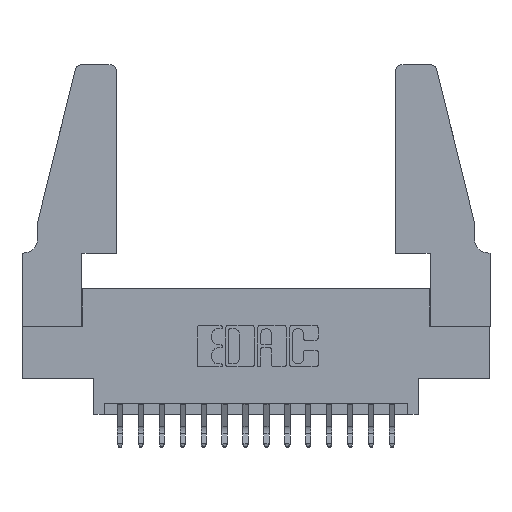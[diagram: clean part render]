
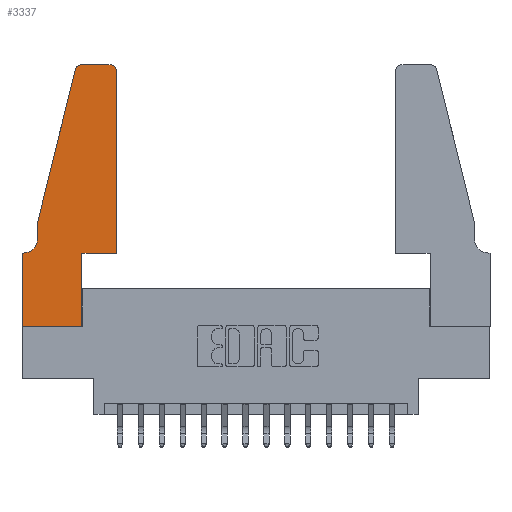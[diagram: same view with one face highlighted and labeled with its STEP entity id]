
A CAD part, top view. The second image highlights one B-rep face of the part: STEP entity #3337.
In plain terms, the highlighted planar face has unit normal (0, 0, 1).
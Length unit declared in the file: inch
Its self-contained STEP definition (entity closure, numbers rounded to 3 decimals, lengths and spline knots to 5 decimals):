
#280 = LINE ( 'NONE', #4821, #7198 ) ;
#361 = DIRECTION ( 'NONE',  ( 1., 0., 0. ) ) ;
#707 = ORIENTED_EDGE ( 'NONE', *, *, #12276, .T. ) ;
#784 = FACE_OUTER_BOUND ( 'NONE', #8492, .T. ) ;
#1114 = EDGE_CURVE ( 'NONE', #12364, #7590, #1750, .T. ) ;
#1328 = DIRECTION ( 'NONE',  ( -0.239, -0.971, 0. ) ) ;
#1640 = CARTESIAN_POINT ( 'NONE',  ( 0.284, 1.25, 0.37 ) ) ;
#1750 = LINE ( 'NONE', #13940, #2628 ) ;
#1906 = AXIS2_PLACEMENT_3D ( 'NONE', #14944, #7088, #16219 ) ;
#1965 = CARTESIAN_POINT ( 'NONE',  ( 0.25487, 1.22718, 0.37 ) ) ;
#2023 = EDGE_CURVE ( 'NONE', #8956, #2541, #10098, .T. ) ;
#2480 = VECTOR ( 'NONE', #1328, 39.37008 ) ;
#2541 = VERTEX_POINT ( 'NONE', #1640 ) ;
#2557 = VERTEX_POINT ( 'NONE', #15580 ) ;
#2628 = VECTOR ( 'NONE', #14097, 39.37008 ) ;
#2693 = ORIENTED_EDGE ( 'NONE', *, *, #15393, .T. ) ;
#2749 = ORIENTED_EDGE ( 'NONE', *, *, #11909, .T. ) ;
#3210 = ORIENTED_EDGE ( 'NONE', *, *, #15504, .T. ) ;
#3218 = VERTEX_POINT ( 'NONE', #13668 ) ;
#3234 = VECTOR ( 'NONE', #13083, 39.37008 ) ;
#3337 = ADVANCED_FACE ( 'NONE', ( #784 ), #7338, .T. ) ;
#3382 = CARTESIAN_POINT ( 'NONE',  ( 0.4505, 1.22, 0.37 ) ) ;
#4008 = CARTESIAN_POINT ( 'NONE',  ( 0.0755, 0.5, 0.37 ) ) ;
#4012 = CARTESIAN_POINT ( 'NONE',  ( 0.4505, 0.35, 0.37 ) ) ;
#4373 = CARTESIAN_POINT ( 'NONE',  ( 0., 0., 0.37 ) ) ;
#4536 = CIRCLE ( 'NONE', #11591, 0.07 ) ;
#4595 = CARTESIAN_POINT ( 'NONE',  ( 0.4505, 0.35, 0.37 ) ) ;
#4716 = VERTEX_POINT ( 'NONE', #3382 ) ;
#4757 = LINE ( 'NONE', #4595, #11326 ) ;
#4821 = CARTESIAN_POINT ( 'NONE',  ( 0., 0., 0.37 ) ) ;
#5519 = ORIENTED_EDGE ( 'NONE', *, *, #11622, .T. ) ;
#5836 = EDGE_CURVE ( 'NONE', #7590, #13595, #280, .T. ) ;
#5894 = CARTESIAN_POINT ( 'NONE',  ( 0.2865, 0.35, 0.37 ) ) ;
#5945 = ORIENTED_EDGE ( 'NONE', *, *, #1114, .T. ) ;
#6180 = DIRECTION ( 'NONE',  ( 0., -1., 0. ) ) ;
#6198 = CARTESIAN_POINT ( 'NONE',  ( 0.2865, 0., 0.37 ) ) ;
#6492 = CARTESIAN_POINT ( 'NONE',  ( 0.4505, 0.35, 0.37 ) ) ;
#6739 = DIRECTION ( 'NONE',  ( 0., -1., 0. ) ) ;
#6822 = ORIENTED_EDGE ( 'NONE', *, *, #9660, .T. ) ;
#7088 = DIRECTION ( 'NONE',  ( 0., 0., 1. ) ) ;
#7198 = VECTOR ( 'NONE', #6180, 39.37008 ) ;
#7237 = LINE ( 'NONE', #8560, #17199 ) ;
#7245 = DIRECTION ( 'NONE',  ( 0., 1., 0. ) ) ;
#7338 = PLANE ( 'NONE',  #9813 ) ;
#7351 = CARTESIAN_POINT ( 'NONE',  ( 0.0055, 0.35, 0.37 ) ) ;
#7442 = ORIENTED_EDGE ( 'NONE', *, *, #8567, .T. ) ;
#7590 = VERTEX_POINT ( 'NONE', #8642 ) ;
#7692 = CARTESIAN_POINT ( 'NONE',  ( 0.0055, 0.42, 0.37 ) ) ;
#7879 = CARTESIAN_POINT ( 'NONE',  ( 0.4205, 1.22, 0.37 ) ) ;
#8240 = CARTESIAN_POINT ( 'NONE',  ( 0.4205, 1.25, 0.37 ) ) ;
#8492 = EDGE_LOOP ( 'NONE', ( #10674, #6822, #3210, #7442, #12555, #5945, #8846, #11333, #707, #5519, #2749, #2693 ) ) ;
#8560 = CARTESIAN_POINT ( 'NONE',  ( 0., 0., 0.37 ) ) ;
#8567 = EDGE_CURVE ( 'NONE', #2557, #3218, #15718, .T. ) ;
#8633 = DIRECTION ( 'NONE',  ( 1., 0., 0. ) ) ;
#8642 = CARTESIAN_POINT ( 'NONE',  ( 0., 0.35, 0.37 ) ) ;
#8846 = ORIENTED_EDGE ( 'NONE', *, *, #5836, .T. ) ;
#8956 = VERTEX_POINT ( 'NONE', #8240 ) ;
#8985 = DIRECTION ( 'NONE',  ( -1., 0., 0. ) ) ;
#9167 = DIRECTION ( 'NONE',  ( 1., 0., 0. ) ) ;
#9660 = EDGE_CURVE ( 'NONE', #2541, #16918, #15879, .T. ) ;
#9726 = DIRECTION ( 'NONE',  ( -1., 0., 0. ) ) ;
#9813 = AXIS2_PLACEMENT_3D ( 'NONE', #9883, #16464, #8633 ) ;
#9883 = CARTESIAN_POINT ( 'NONE',  ( 0., 0.35, 0.37 ) ) ;
#10098 = LINE ( 'NONE', #14722, #12789 ) ;
#10674 = ORIENTED_EDGE ( 'NONE', *, *, #2023, .T. ) ;
#10713 = CARTESIAN_POINT ( 'NONE',  ( 0.0755, 0.5, 0.37 ) ) ;
#11087 = EDGE_CURVE ( 'NONE', #13595, #15828, #7237, .T. ) ;
#11326 = VECTOR ( 'NONE', #361, 39.37008 ) ;
#11333 = ORIENTED_EDGE ( 'NONE', *, *, #11087, .T. ) ;
#11511 = VECTOR ( 'NONE', #7245, 39.37008 ) ;
#11591 = AXIS2_PLACEMENT_3D ( 'NONE', #7692, #16810, #8985 ) ;
#11622 = EDGE_CURVE ( 'NONE', #11815, #13387, #4757, .T. ) ;
#11815 = VERTEX_POINT ( 'NONE', #14209 ) ;
#11834 = EDGE_CURVE ( 'NONE', #3218, #12364, #4536, .T. ) ;
#11909 = EDGE_CURVE ( 'NONE', #13387, #4716, #14258, .T. ) ;
#11935 = LINE ( 'NONE', #5894, #11511 ) ;
#12052 = CIRCLE ( 'NONE', #14227, 0.03 ) ;
#12214 = VECTOR ( 'NONE', #6739, 39.37008 ) ;
#12276 = EDGE_CURVE ( 'NONE', #15828, #11815, #11935, .T. ) ;
#12364 = VERTEX_POINT ( 'NONE', #7351 ) ;
#12517 = DIRECTION ( 'NONE',  ( 1., 0., 0. ) ) ;
#12555 = ORIENTED_EDGE ( 'NONE', *, *, #11834, .T. ) ;
#12789 = VECTOR ( 'NONE', #9726, 39.37008 ) ;
#13083 = DIRECTION ( 'NONE',  ( 0., 1., 0. ) ) ;
#13387 = VERTEX_POINT ( 'NONE', #4012 ) ;
#13595 = VERTEX_POINT ( 'NONE', #4373 ) ;
#13668 = CARTESIAN_POINT ( 'NONE',  ( 0.0755, 0.42, 0.37 ) ) ;
#13940 = CARTESIAN_POINT ( 'NONE',  ( 0.0755, 0.35, 0.37 ) ) ;
#14097 = DIRECTION ( 'NONE',  ( -1., 0., 0. ) ) ;
#14209 = CARTESIAN_POINT ( 'NONE',  ( 0.2865, 0.35, 0.37 ) ) ;
#14227 = AXIS2_PLACEMENT_3D ( 'NONE', #7879, #16989, #9167 ) ;
#14258 = LINE ( 'NONE', #6492, #3234 ) ;
#14722 = CARTESIAN_POINT ( 'NONE',  ( 0.2605, 1.25, 0.37 ) ) ;
#14944 = CARTESIAN_POINT ( 'NONE',  ( 0.284, 1.22, 0.37 ) ) ;
#15393 = EDGE_CURVE ( 'NONE', #4716, #8956, #12052, .T. ) ;
#15504 = EDGE_CURVE ( 'NONE', #16918, #2557, #16160, .T. ) ;
#15580 = CARTESIAN_POINT ( 'NONE',  ( 0.0755, 0.5, 0.37 ) ) ;
#15718 = LINE ( 'NONE', #4008, #12214 ) ;
#15828 = VERTEX_POINT ( 'NONE', #6198 ) ;
#15879 = CIRCLE ( 'NONE', #1906, 0.03 ) ;
#16160 = LINE ( 'NONE', #10713, #2480 ) ;
#16219 = DIRECTION ( 'NONE',  ( 1., 0., 0. ) ) ;
#16464 = DIRECTION ( 'NONE',  ( 0., 0., 1. ) ) ;
#16810 = DIRECTION ( 'NONE',  ( 0., 0., -1. ) ) ;
#16918 = VERTEX_POINT ( 'NONE', #1965 ) ;
#16989 = DIRECTION ( 'NONE',  ( 0., 0., 1. ) ) ;
#17199 = VECTOR ( 'NONE', #12517, 39.37008 ) ;
